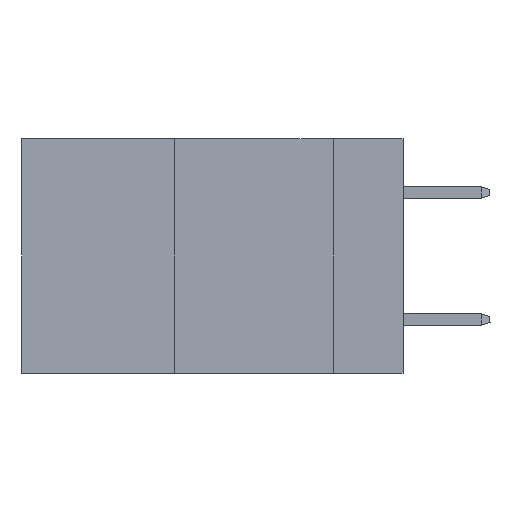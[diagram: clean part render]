
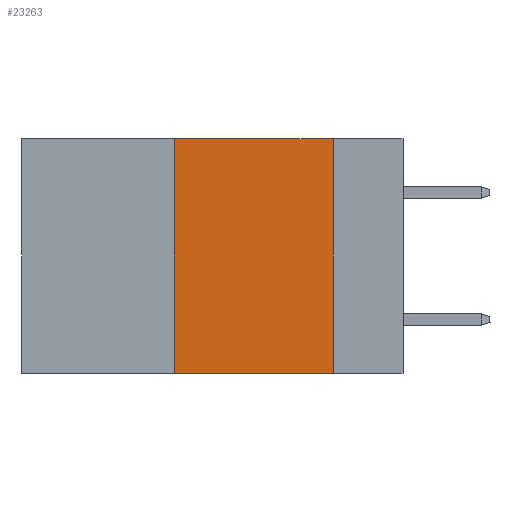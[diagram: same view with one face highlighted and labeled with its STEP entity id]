
A CAD part, left-side view. The second image highlights one B-rep face of the part: STEP entity #23263.
In plain terms, the highlighted planar face has unit normal (-1, 0, 0).
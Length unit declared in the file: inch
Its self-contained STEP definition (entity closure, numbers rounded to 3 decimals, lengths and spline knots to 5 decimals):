
#520 = DIRECTION ( 'NONE',  ( 0., 0., 1. ) ) ;
#900 = EDGE_CURVE ( 'NONE', #20200, #8813, #10480, .T. ) ;
#1725 = DIRECTION ( 'NONE',  ( 0., 0., -1. ) ) ;
#1804 = ORIENTED_EDGE ( 'NONE', *, *, #10512, .F. ) ;
#3549 = CARTESIAN_POINT ( 'NONE',  ( 0., 0.6, 0. ) ) ;
#3587 = ORIENTED_EDGE ( 'NONE', *, *, #900, .F. ) ;
#4332 = CARTESIAN_POINT ( 'NONE',  ( 0., 0.36, -0.37 ) ) ;
#4812 = VECTOR ( 'NONE', #520, 39.37008 ) ;
#5269 = PLANE ( 'NONE',  #19525 ) ;
#5320 = LINE ( 'NONE', #9059, #15233 ) ;
#6547 = VERTEX_POINT ( 'NONE', #4332 ) ;
#6703 = ORIENTED_EDGE ( 'NONE', *, *, #18131, .F. ) ;
#8813 = VERTEX_POINT ( 'NONE', #20909 ) ;
#9059 = CARTESIAN_POINT ( 'NONE',  ( 0., 0.6, 0. ) ) ;
#9972 = CARTESIAN_POINT ( 'NONE',  ( 0., 0.36, 0. ) ) ;
#10480 = LINE ( 'NONE', #12538, #13446 ) ;
#10512 = EDGE_CURVE ( 'NONE', #6547, #19481, #17478, .T. ) ;
#10601 = DIRECTION ( 'NONE',  ( 0., 0., -1. ) ) ;
#10932 = DIRECTION ( 'NONE',  ( 1., 0., 0. ) ) ;
#11771 = EDGE_CURVE ( 'NONE', #6547, #8813, #19974, .T. ) ;
#12538 = CARTESIAN_POINT ( 'NONE',  ( 0., 0.11, 0. ) ) ;
#12580 = DIRECTION ( 'NONE',  ( 0., -1., 0. ) ) ;
#12949 = CARTESIAN_POINT ( 'NONE',  ( 0., 0.36, 0. ) ) ;
#13011 = FACE_OUTER_BOUND ( 'NONE', #17741, .T. ) ;
#13446 = VECTOR ( 'NONE', #10601, 39.37008 ) ;
#14652 = DIRECTION ( 'NONE',  ( 0., -1., 0. ) ) ;
#15233 = VECTOR ( 'NONE', #14652, 39.37008 ) ;
#17478 = LINE ( 'NONE', #9972, #4812 ) ;
#17741 = EDGE_LOOP ( 'NONE', ( #3587, #6703, #1804, #19886 ) ) ;
#18131 = EDGE_CURVE ( 'NONE', #19481, #20200, #5320, .T. ) ;
#19481 = VERTEX_POINT ( 'NONE', #12949 ) ;
#19525 = AXIS2_PLACEMENT_3D ( 'NONE', #3549, #10932, #1725 ) ;
#19886 = ORIENTED_EDGE ( 'NONE', *, *, #11771, .T. ) ;
#19974 = LINE ( 'NONE', #20433, #21045 ) ;
#20200 = VERTEX_POINT ( 'NONE', #21631 ) ;
#20433 = CARTESIAN_POINT ( 'NONE',  ( 0., 0.6, -0.37 ) ) ;
#20909 = CARTESIAN_POINT ( 'NONE',  ( 0., 0.11, -0.37 ) ) ;
#21045 = VECTOR ( 'NONE', #12580, 39.37008 ) ;
#21631 = CARTESIAN_POINT ( 'NONE',  ( 0., 0.11, 0. ) ) ;
#23263 = ADVANCED_FACE ( 'NONE', ( #13011 ), #5269, .F. ) ;
